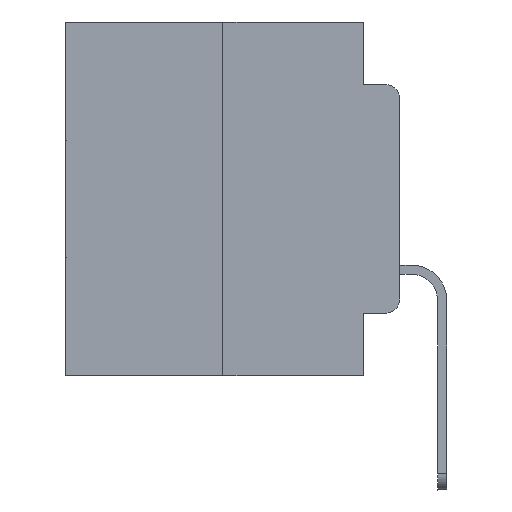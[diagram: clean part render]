
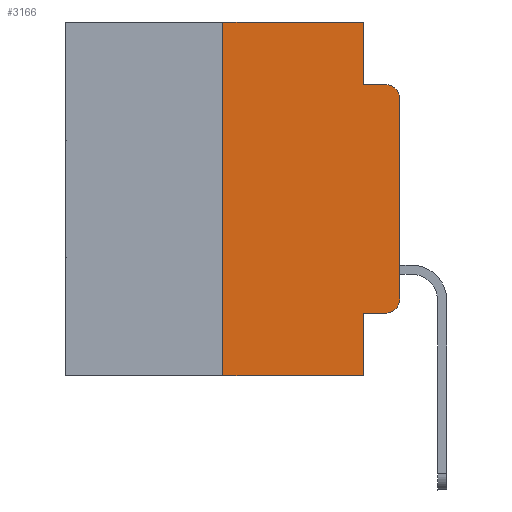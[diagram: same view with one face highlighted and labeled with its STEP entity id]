
A CAD part, left-side view. The second image highlights one B-rep face of the part: STEP entity #3166.
In plain terms, the highlighted planar face has unit normal (-1, 0, 0).
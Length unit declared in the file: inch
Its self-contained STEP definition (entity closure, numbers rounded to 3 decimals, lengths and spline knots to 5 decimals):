
#216 = VECTOR ( 'NONE', #7215, 39.37008 ) ;
#534 = VERTEX_POINT ( 'NONE', #13202 ) ;
#591 = LINE ( 'NONE', #17087, #4311 ) ;
#657 = CARTESIAN_POINT ( 'NONE',  ( 0., 0.051, -0.0885 ) ) ;
#727 = CARTESIAN_POINT ( 'NONE',  ( 0., 0.051, -0.5 ) ) ;
#1057 = CARTESIAN_POINT ( 'NONE',  ( 0., 0.473, -0.5 ) ) ;
#1551 = DIRECTION ( 'NONE',  ( -1., 0., 0. ) ) ;
#2737 = DIRECTION ( 'NONE',  ( 0., 0., -1. ) ) ;
#3166 = ADVANCED_FACE ( 'NONE', ( #18973 ), #12709, .F. ) ;
#3677 = CARTESIAN_POINT ( 'NONE',  ( 0., 0.25, -0.5 ) ) ;
#4022 = DIRECTION ( 'NONE',  ( 0., 0., -1. ) ) ;
#4037 = DIRECTION ( 'NONE',  ( 0., -1., 0. ) ) ;
#4107 = EDGE_CURVE ( 'NONE', #15352, #23732, #19823, .T. ) ;
#4311 = VECTOR ( 'NONE', #17365, 39.37008 ) ;
#4797 = DIRECTION ( 'NONE',  ( -1., 0., 0. ) ) ;
#5666 = VERTEX_POINT ( 'NONE', #16094 ) ;
#5737 = CARTESIAN_POINT ( 'NONE',  ( 0., 0.02, -0.0885 ) ) ;
#6119 = VECTOR ( 'NONE', #25769, 39.37008 ) ;
#6344 = LINE ( 'NONE', #22707, #8573 ) ;
#6444 = EDGE_CURVE ( 'NONE', #15352, #18420, #19740, .T. ) ;
#6568 = LINE ( 'NONE', #8490, #23819 ) ;
#7077 = ORIENTED_EDGE ( 'NONE', *, *, #8307, .F. ) ;
#7123 = EDGE_CURVE ( 'NONE', #534, #9946, #16021, .T. ) ;
#7130 = CARTESIAN_POINT ( 'NONE',  ( 0., 0.25, 0. ) ) ;
#7215 = DIRECTION ( 'NONE',  ( 0., -1., 0. ) ) ;
#7233 = ORIENTED_EDGE ( 'NONE', *, *, #16330, .T. ) ;
#7434 = DIRECTION ( 'NONE',  ( 0., 0., 1. ) ) ;
#7502 = VERTEX_POINT ( 'NONE', #657 ) ;
#7797 = EDGE_LOOP ( 'NONE', ( #15853, #26106, #20850, #13335, #17581, #19546, #20977, #7077, #7233, #17965 ) ) ;
#8122 = VERTEX_POINT ( 'NONE', #19442 ) ;
#8307 = EDGE_CURVE ( 'NONE', #5666, #18420, #20784, .T. ) ;
#8490 = CARTESIAN_POINT ( 'NONE',  ( 0., 0.051, -0.4115 ) ) ;
#8573 = VECTOR ( 'NONE', #4037, 39.37008 ) ;
#8639 = CARTESIAN_POINT ( 'NONE',  ( 0., 0.473, 0. ) ) ;
#8986 = EDGE_CURVE ( 'NONE', #8122, #534, #9141, .T. ) ;
#9141 = LINE ( 'NONE', #17426, #6119 ) ;
#9946 = VERTEX_POINT ( 'NONE', #5737 ) ;
#10138 = CARTESIAN_POINT ( 'NONE',  ( 0., 0.051, 0. ) ) ;
#10426 = CARTESIAN_POINT ( 'NONE',  ( 0., 0.051, 0. ) ) ;
#12709 = PLANE ( 'NONE',  #26206 ) ;
#13202 = CARTESIAN_POINT ( 'NONE',  ( 0., 0., -0.1085 ) ) ;
#13309 = CARTESIAN_POINT ( 'NONE',  ( 0., 0.051, 0. ) ) ;
#13335 = ORIENTED_EDGE ( 'NONE', *, *, #24652, .F. ) ;
#13422 = CARTESIAN_POINT ( 'NONE',  ( 0., 0.02, -0.4115 ) ) ;
#14149 = DIRECTION ( 'NONE',  ( 0., 0., -1. ) ) ;
#14664 = EDGE_CURVE ( 'NONE', #24548, #8122, #15864, .T. ) ;
#15352 = VERTEX_POINT ( 'NONE', #3677 ) ;
#15853 = ORIENTED_EDGE ( 'NONE', *, *, #8986, .T. ) ;
#15864 = CIRCLE ( 'NONE', #20234, 0.02 ) ;
#16021 = CIRCLE ( 'NONE', #19523, 0.02 ) ;
#16094 = CARTESIAN_POINT ( 'NONE',  ( 0., 0.051, -0.4115 ) ) ;
#16330 = EDGE_CURVE ( 'NONE', #5666, #24548, #6568, .T. ) ;
#16524 = VECTOR ( 'NONE', #4022, 39.37008 ) ;
#17087 = CARTESIAN_POINT ( 'NONE',  ( 0., 0.473, 0. ) ) ;
#17365 = DIRECTION ( 'NONE',  ( 0., -1., 0. ) ) ;
#17426 = CARTESIAN_POINT ( 'NONE',  ( 0., 0., 0. ) ) ;
#17581 = ORIENTED_EDGE ( 'NONE', *, *, #18456, .F. ) ;
#17965 = ORIENTED_EDGE ( 'NONE', *, *, #14664, .T. ) ;
#18014 = VECTOR ( 'NONE', #18436, 39.37008 ) ;
#18420 = VERTEX_POINT ( 'NONE', #727 ) ;
#18436 = DIRECTION ( 'NONE',  ( 0., 0., -1. ) ) ;
#18456 = EDGE_CURVE ( 'NONE', #23732, #22795, #591, .T. ) ;
#18973 = FACE_OUTER_BOUND ( 'NONE', #7797, .T. ) ;
#19111 = DIRECTION ( 'NONE',  ( 1., 0., 0. ) ) ;
#19442 = CARTESIAN_POINT ( 'NONE',  ( 0., 0., -0.3915 ) ) ;
#19523 = AXIS2_PLACEMENT_3D ( 'NONE', #23469, #4797, #2737 ) ;
#19546 = ORIENTED_EDGE ( 'NONE', *, *, #4107, .F. ) ;
#19740 = LINE ( 'NONE', #1057, #216 ) ;
#19823 = LINE ( 'NONE', #26385, #21904 ) ;
#20229 = CARTESIAN_POINT ( 'NONE',  ( 0., 0.02, -0.3915 ) ) ;
#20234 = AXIS2_PLACEMENT_3D ( 'NONE', #20229, #1551, #26672 ) ;
#20784 = LINE ( 'NONE', #10426, #16524 ) ;
#20850 = ORIENTED_EDGE ( 'NONE', *, *, #26598, .F. ) ;
#20977 = ORIENTED_EDGE ( 'NONE', *, *, #6444, .T. ) ;
#21904 = VECTOR ( 'NONE', #7434, 39.37008 ) ;
#22707 = CARTESIAN_POINT ( 'NONE',  ( 0., 0.051, -0.0885 ) ) ;
#22795 = VERTEX_POINT ( 'NONE', #13309 ) ;
#22802 = LINE ( 'NONE', #10138, #18014 ) ;
#23469 = CARTESIAN_POINT ( 'NONE',  ( 0., 0.02, -0.1085 ) ) ;
#23732 = VERTEX_POINT ( 'NONE', #7130 ) ;
#23819 = VECTOR ( 'NONE', #24992, 39.37008 ) ;
#24548 = VERTEX_POINT ( 'NONE', #13422 ) ;
#24652 = EDGE_CURVE ( 'NONE', #22795, #7502, #22802, .T. ) ;
#24992 = DIRECTION ( 'NONE',  ( 0., -1., 0. ) ) ;
#25769 = DIRECTION ( 'NONE',  ( 0., 0., 1. ) ) ;
#26106 = ORIENTED_EDGE ( 'NONE', *, *, #7123, .T. ) ;
#26206 = AXIS2_PLACEMENT_3D ( 'NONE', #8639, #19111, #14149 ) ;
#26385 = CARTESIAN_POINT ( 'NONE',  ( 0., 0.25, 0. ) ) ;
#26598 = EDGE_CURVE ( 'NONE', #7502, #9946, #6344, .T. ) ;
#26672 = DIRECTION ( 'NONE',  ( 0., 0., -1. ) ) ;
